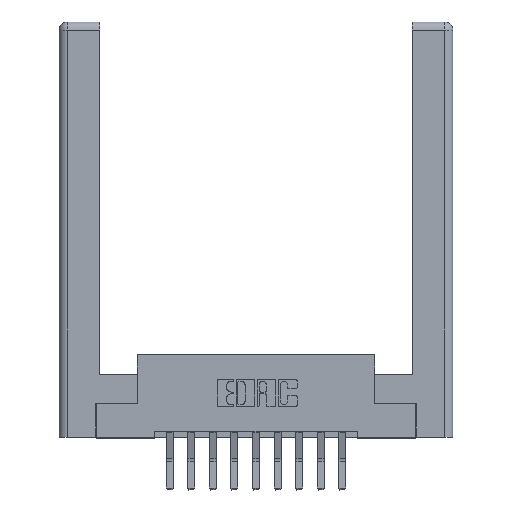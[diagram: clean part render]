
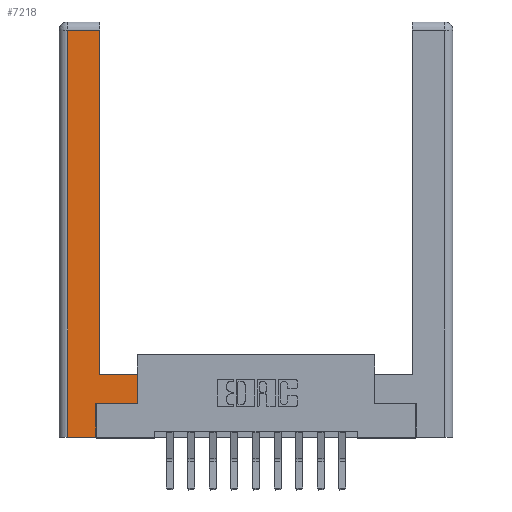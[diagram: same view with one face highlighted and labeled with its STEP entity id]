
A CAD part, top view. The second image highlights one B-rep face of the part: STEP entity #7218.
In plain terms, the highlighted planar face has unit normal (0, 0, 1).
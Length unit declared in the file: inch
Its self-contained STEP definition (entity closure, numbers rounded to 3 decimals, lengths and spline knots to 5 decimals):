
#236 = CARTESIAN_POINT ( 'NONE',  ( 0.265, 0.245, 0. ) ) ;
#736 = CARTESIAN_POINT ( 'NONE',  ( 0.0615, 2.94, 0. ) ) ;
#912 = EDGE_CURVE ( 'NONE', #12899, #10733, #3911, .T. ) ;
#1011 = VECTOR ( 'NONE', #10038, 39.37008 ) ;
#1037 = VECTOR ( 'NONE', #7917, 39.37008 ) ;
#1077 = CARTESIAN_POINT ( 'NONE',  ( 0., 0., 0. ) ) ;
#1144 = CARTESIAN_POINT ( 'NONE',  ( 0.295, 0.45, 0. ) ) ;
#1285 = DIRECTION ( 'NONE',  ( 0., 0., -1. ) ) ;
#1443 = CARTESIAN_POINT ( 'NONE',  ( 0.0615, 0., 0. ) ) ;
#1473 = DIRECTION ( 'NONE',  ( -1., 0., 0. ) ) ;
#1577 = ORIENTED_EDGE ( 'NONE', *, *, #1654, .T. ) ;
#1654 = EDGE_CURVE ( 'NONE', #13406, #3730, #2722, .T. ) ;
#2166 = LINE ( 'NONE', #236, #10061 ) ;
#2228 = EDGE_LOOP ( 'NONE', ( #2763, #8550, #5083, #4385, #8721, #8664, #1577, #12894 ) ) ;
#2525 = CARTESIAN_POINT ( 'NONE',  ( 0.565, 0.45, 0. ) ) ;
#2722 = LINE ( 'NONE', #2525, #1011 ) ;
#2763 = ORIENTED_EDGE ( 'NONE', *, *, #11537, .T. ) ;
#2850 = LINE ( 'NONE', #736, #3195 ) ;
#3195 = VECTOR ( 'NONE', #12649, 39.37008 ) ;
#3392 = VECTOR ( 'NONE', #10531, 39.37008 ) ;
#3562 = VECTOR ( 'NONE', #12233, 39.37008 ) ;
#3730 = VERTEX_POINT ( 'NONE', #13258 ) ;
#3814 = VECTOR ( 'NONE', #10362, 39.37008 ) ;
#3911 = LINE ( 'NONE', #1443, #1037 ) ;
#4054 = CARTESIAN_POINT ( 'NONE',  ( 0.0615, 0., 0. ) ) ;
#4385 = ORIENTED_EDGE ( 'NONE', *, *, #10450, .T. ) ;
#4594 = LINE ( 'NONE', #8954, #3562 ) ;
#4806 = VECTOR ( 'NONE', #7677, 39.37008 ) ;
#4882 = EDGE_CURVE ( 'NONE', #3730, #9955, #8204, .T. ) ;
#4971 = CARTESIAN_POINT ( 'NONE',  ( 0.295, 2.94, 0. ) ) ;
#5055 = VERTEX_POINT ( 'NONE', #11098 ) ;
#5083 = ORIENTED_EDGE ( 'NONE', *, *, #912, .T. ) ;
#5638 = CARTESIAN_POINT ( 'NONE',  ( 0.0615, 2.94, 0. ) ) ;
#5991 = CARTESIAN_POINT ( 'NONE',  ( 0.295, 0.45, 0. ) ) ;
#6616 = CARTESIAN_POINT ( 'NONE',  ( 0.265, 0., 0. ) ) ;
#7197 = CARTESIAN_POINT ( 'NONE',  ( 0.265, 0.245, 0. ) ) ;
#7208 = EDGE_CURVE ( 'NONE', #7385, #12899, #2850, .T. ) ;
#7218 = ADVANCED_FACE ( 'NONE', ( #11075 ), #10545, .F. ) ;
#7385 = VERTEX_POINT ( 'NONE', #4971 ) ;
#7556 = AXIS2_PLACEMENT_3D ( 'NONE', #1077, #1285, #1473 ) ;
#7677 = DIRECTION ( 'NONE',  ( 1., 0., 0. ) ) ;
#7730 = EDGE_CURVE ( 'NONE', #5055, #12501, #2166, .T. ) ;
#7917 = DIRECTION ( 'NONE',  ( 0., -1., 0. ) ) ;
#8204 = LINE ( 'NONE', #5991, #3814 ) ;
#8340 = CARTESIAN_POINT ( 'NONE',  ( 0.565, 0.245, 0. ) ) ;
#8550 = ORIENTED_EDGE ( 'NONE', *, *, #7208, .T. ) ;
#8664 = ORIENTED_EDGE ( 'NONE', *, *, #12508, .T. ) ;
#8721 = ORIENTED_EDGE ( 'NONE', *, *, #7730, .T. ) ;
#8954 = CARTESIAN_POINT ( 'NONE',  ( 0.295, 3., 0. ) ) ;
#9096 = LINE ( 'NONE', #8340, #3392 ) ;
#9955 = VERTEX_POINT ( 'NONE', #1144 ) ;
#10038 = DIRECTION ( 'NONE',  ( 0., 1., 0. ) ) ;
#10061 = VECTOR ( 'NONE', #12118, 39.37008 ) ;
#10362 = DIRECTION ( 'NONE',  ( -1., 0., 0. ) ) ;
#10450 = EDGE_CURVE ( 'NONE', #10733, #5055, #13712, .T. ) ;
#10531 = DIRECTION ( 'NONE',  ( 1., 0., 0. ) ) ;
#10545 = PLANE ( 'NONE',  #7556 ) ;
#10733 = VERTEX_POINT ( 'NONE', #4054 ) ;
#10777 = CARTESIAN_POINT ( 'NONE',  ( 0.565, 0.245, 0. ) ) ;
#11075 = FACE_OUTER_BOUND ( 'NONE', #2228, .T. ) ;
#11098 = CARTESIAN_POINT ( 'NONE',  ( 0.265, 0., 0. ) ) ;
#11537 = EDGE_CURVE ( 'NONE', #9955, #7385, #4594, .T. ) ;
#12118 = DIRECTION ( 'NONE',  ( 0., 1., 0. ) ) ;
#12233 = DIRECTION ( 'NONE',  ( 0., 1., 0. ) ) ;
#12501 = VERTEX_POINT ( 'NONE', #7197 ) ;
#12508 = EDGE_CURVE ( 'NONE', #12501, #13406, #9096, .T. ) ;
#12649 = DIRECTION ( 'NONE',  ( -1., 0., 0. ) ) ;
#12894 = ORIENTED_EDGE ( 'NONE', *, *, #4882, .T. ) ;
#12899 = VERTEX_POINT ( 'NONE', #5638 ) ;
#13258 = CARTESIAN_POINT ( 'NONE',  ( 0.565, 0.45, 0. ) ) ;
#13406 = VERTEX_POINT ( 'NONE', #10777 ) ;
#13712 = LINE ( 'NONE', #6616, #4806 ) ;
